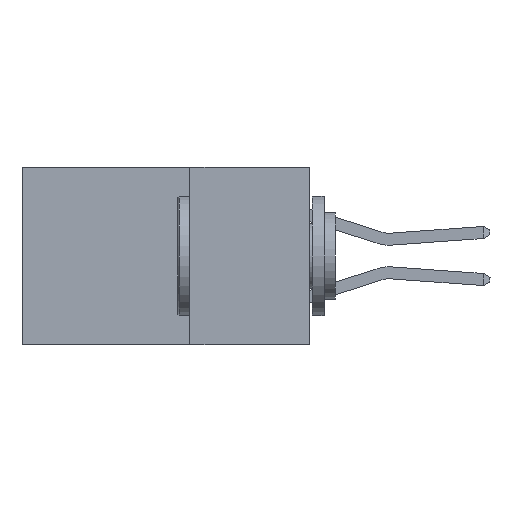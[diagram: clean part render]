
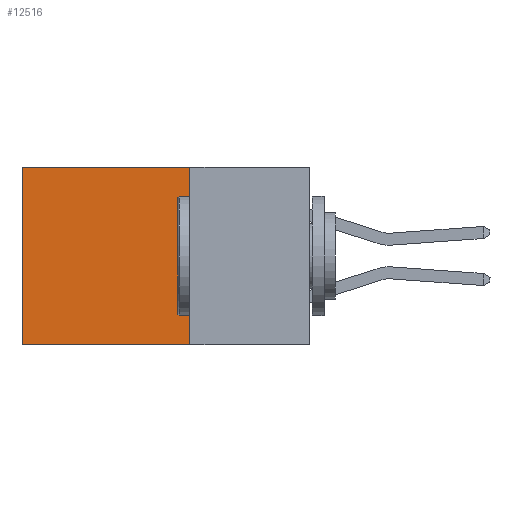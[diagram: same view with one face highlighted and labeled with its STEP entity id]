
A CAD part, left-side view. The second image highlights one B-rep face of the part: STEP entity #12516.
In plain terms, the highlighted planar face has unit normal (-1, 0, 0).
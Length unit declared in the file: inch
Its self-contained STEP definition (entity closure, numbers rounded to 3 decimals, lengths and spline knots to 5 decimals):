
#87 = EDGE_CURVE ( 'NONE', #15284, #15311, #4621, .T. ) ;
#455 = CARTESIAN_POINT ( 'NONE',  ( 0.298, 0.25, -0.37 ) ) ;
#633 = DIRECTION ( 'NONE',  ( 0., 1., 0. ) ) ;
#2291 = CARTESIAN_POINT ( 'NONE',  ( 0.298, 0.6, 0. ) ) ;
#2905 = VECTOR ( 'NONE', #7587, 39.37008 ) ;
#3359 = ORIENTED_EDGE ( 'NONE', *, *, #15064, .F. ) ;
#3384 = CARTESIAN_POINT ( 'NONE',  ( 0.298, 0.25, 0. ) ) ;
#3406 = DIRECTION ( 'NONE',  ( 0., 0., -1. ) ) ;
#3581 = ORIENTED_EDGE ( 'NONE', *, *, #87, .T. ) ;
#3658 = ORIENTED_EDGE ( 'NONE', *, *, #7642, .F. ) ;
#3972 = CARTESIAN_POINT ( 'NONE',  ( 0.298, 0.25, -0.37 ) ) ;
#4621 = LINE ( 'NONE', #2291, #2905 ) ;
#4914 = CARTESIAN_POINT ( 'NONE',  ( 0.298, 0.25, 0. ) ) ;
#5296 = ORIENTED_EDGE ( 'NONE', *, *, #9892, .T. ) ;
#5375 = LINE ( 'NONE', #4914, #8588 ) ;
#6201 = DIRECTION ( 'NONE',  ( 0., 1., 0. ) ) ;
#7218 = VERTEX_POINT ( 'NONE', #3972 ) ;
#7579 = DIRECTION ( 'NONE',  ( 1., 0., 0. ) ) ;
#7582 = CARTESIAN_POINT ( 'NONE',  ( 0.298, 0.25, 0. ) ) ;
#7587 = DIRECTION ( 'NONE',  ( 0., 0., -1. ) ) ;
#7642 = EDGE_CURVE ( 'NONE', #7218, #15311, #16534, .T. ) ;
#8545 = AXIS2_PLACEMENT_3D ( 'NONE', #3384, #7579, #13006 ) ;
#8588 = VECTOR ( 'NONE', #3406, 39.37008 ) ;
#9733 = EDGE_LOOP ( 'NONE', ( #3581, #3658, #3359, #5296 ) ) ;
#9892 = EDGE_CURVE ( 'NONE', #13015, #15284, #16466, .T. ) ;
#10901 = CARTESIAN_POINT ( 'NONE',  ( 0.298, 0.6, -0.37 ) ) ;
#11242 = CARTESIAN_POINT ( 'NONE',  ( 0.298, 0.25, 0. ) ) ;
#11873 = PLANE ( 'NONE',  #8545 ) ;
#12233 = CARTESIAN_POINT ( 'NONE',  ( 0.298, 0.6, 0. ) ) ;
#12516 = ADVANCED_FACE ( 'NONE', ( #13804 ), #11873, .F. ) ;
#13006 = DIRECTION ( 'NONE',  ( 0., 0., -1. ) ) ;
#13015 = VERTEX_POINT ( 'NONE', #11242 ) ;
#13804 = FACE_OUTER_BOUND ( 'NONE', #9733, .T. ) ;
#15064 = EDGE_CURVE ( 'NONE', #13015, #7218, #5375, .T. ) ;
#15165 = VECTOR ( 'NONE', #6201, 39.37008 ) ;
#15284 = VERTEX_POINT ( 'NONE', #12233 ) ;
#15311 = VERTEX_POINT ( 'NONE', #10901 ) ;
#16466 = LINE ( 'NONE', #7582, #15165 ) ;
#16534 = LINE ( 'NONE', #455, #17607 ) ;
#17607 = VECTOR ( 'NONE', #633, 39.37008 ) ;
